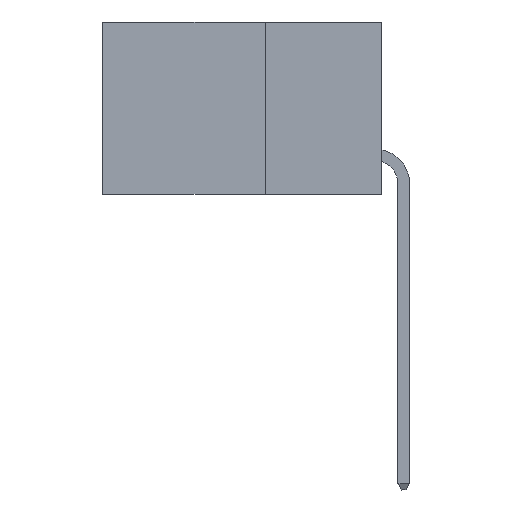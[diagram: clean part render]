
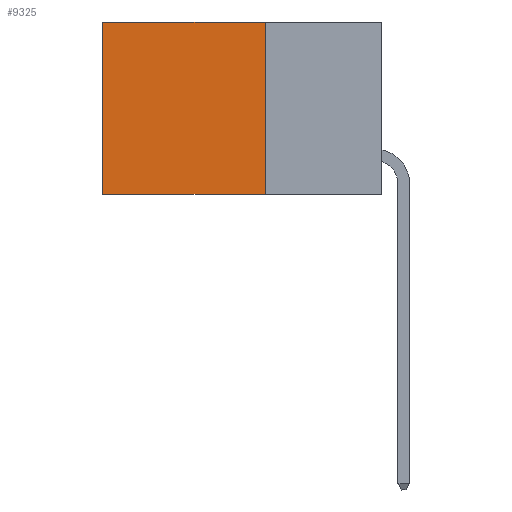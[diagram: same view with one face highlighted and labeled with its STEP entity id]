
A CAD part, left-side view. The second image highlights one B-rep face of the part: STEP entity #9325.
In plain terms, the highlighted planar face has unit normal (-1, 0, 0).
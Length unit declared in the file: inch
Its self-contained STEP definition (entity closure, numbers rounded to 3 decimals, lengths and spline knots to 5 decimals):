
#566 = LINE ( 'NONE', #18030, #13675 ) ;
#571 = VECTOR ( 'NONE', #30571, 39.37008 ) ;
#1435 = DIRECTION ( 'NONE',  ( 0., 0., -1. ) ) ;
#1623 = LINE ( 'NONE', #21800, #14732 ) ;
#4016 = DIRECTION ( 'NONE',  ( 0., 1., 0. ) ) ;
#5566 = VERTEX_POINT ( 'NONE', #35174 ) ;
#9325 = ADVANCED_FACE ( 'NONE', ( #31353 ), #34704, .F. ) ;
#10699 = AXIS2_PLACEMENT_3D ( 'NONE', #31945, #18229, #1435 ) ;
#11530 = VERTEX_POINT ( 'NONE', #13105 ) ;
#12545 = EDGE_CURVE ( 'NONE', #25849, #11530, #33771, .T. ) ;
#13105 = CARTESIAN_POINT ( 'NONE',  ( 0.2875, 0.6, -0.37 ) ) ;
#13675 = VECTOR ( 'NONE', #4016, 39.37008 ) ;
#14732 = VECTOR ( 'NONE', #30047, 39.37008 ) ;
#15480 = ORIENTED_EDGE ( 'NONE', *, *, #32617, .F. ) ;
#18030 = CARTESIAN_POINT ( 'NONE',  ( 0.2875, 0.25, -0.37 ) ) ;
#18229 = DIRECTION ( 'NONE',  ( 1., 0., 0. ) ) ;
#18644 = EDGE_LOOP ( 'NONE', ( #33650, #23699, #15480, #33493 ) ) ;
#19430 = VERTEX_POINT ( 'NONE', #27533 ) ;
#20841 = EDGE_CURVE ( 'NONE', #19430, #25849, #1623, .T. ) ;
#21800 = CARTESIAN_POINT ( 'NONE',  ( 0.2875, 0.25, 0. ) ) ;
#23699 = ORIENTED_EDGE ( 'NONE', *, *, #23743, .F. ) ;
#23743 = EDGE_CURVE ( 'NONE', #5566, #11530, #566, .T. ) ;
#23846 = LINE ( 'NONE', #33202, #571 ) ;
#23953 = CARTESIAN_POINT ( 'NONE',  ( 0.2875, 0.6, 0. ) ) ;
#25680 = VECTOR ( 'NONE', #29187, 39.37008 ) ;
#25849 = VERTEX_POINT ( 'NONE', #23953 ) ;
#27533 = CARTESIAN_POINT ( 'NONE',  ( 0.2875, 0.25, 0. ) ) ;
#29187 = DIRECTION ( 'NONE',  ( 0., 0., -1. ) ) ;
#30047 = DIRECTION ( 'NONE',  ( 0., 1., 0. ) ) ;
#30571 = DIRECTION ( 'NONE',  ( 0., 0., -1. ) ) ;
#31353 = FACE_OUTER_BOUND ( 'NONE', #18644, .T. ) ;
#31906 = CARTESIAN_POINT ( 'NONE',  ( 0.2875, 0.6, 0. ) ) ;
#31945 = CARTESIAN_POINT ( 'NONE',  ( 0.2875, 0.25, 0. ) ) ;
#32617 = EDGE_CURVE ( 'NONE', #19430, #5566, #23846, .T. ) ;
#33202 = CARTESIAN_POINT ( 'NONE',  ( 0.2875, 0.25, 0. ) ) ;
#33493 = ORIENTED_EDGE ( 'NONE', *, *, #20841, .T. ) ;
#33650 = ORIENTED_EDGE ( 'NONE', *, *, #12545, .T. ) ;
#33771 = LINE ( 'NONE', #31906, #25680 ) ;
#34704 = PLANE ( 'NONE',  #10699 ) ;
#35174 = CARTESIAN_POINT ( 'NONE',  ( 0.2875, 0.25, -0.37 ) ) ;
